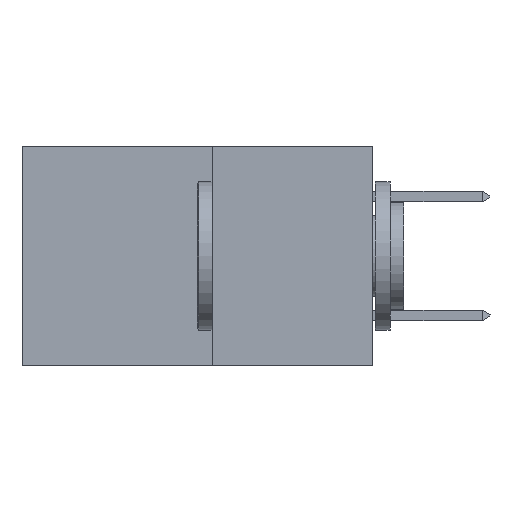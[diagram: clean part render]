
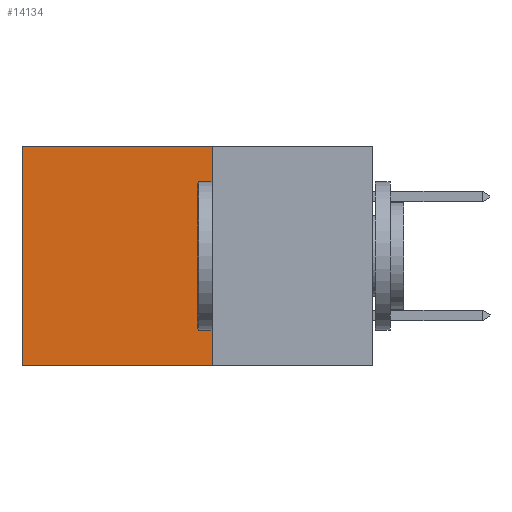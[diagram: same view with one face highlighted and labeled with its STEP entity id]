
A CAD part, left-side view. The second image highlights one B-rep face of the part: STEP entity #14134.
In plain terms, the highlighted planar face has unit normal (-1, 0, 0).
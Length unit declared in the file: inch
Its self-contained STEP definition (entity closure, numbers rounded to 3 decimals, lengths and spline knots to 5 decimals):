
#469 = EDGE_LOOP ( 'NONE', ( #17159, #15991, #15675, #19492 ) ) ;
#588 = EDGE_CURVE ( 'NONE', #6315, #1930, #10557, .T. ) ;
#1930 = VERTEX_POINT ( 'NONE', #6053 ) ;
#3744 = DIRECTION ( 'NONE',  ( 1., 0., 0. ) ) ;
#4343 = VERTEX_POINT ( 'NONE', #8386 ) ;
#6053 = CARTESIAN_POINT ( 'NONE',  ( 0.277, 0.59, 0. ) ) ;
#6055 = VECTOR ( 'NONE', #16469, 39.37008 ) ;
#6247 = EDGE_CURVE ( 'NONE', #1930, #4343, #13779, .T. ) ;
#6263 = EDGE_CURVE ( 'NONE', #6315, #13276, #17851, .T. ) ;
#6315 = VERTEX_POINT ( 'NONE', #9423 ) ;
#6545 = CARTESIAN_POINT ( 'NONE',  ( 0.277, 0.27, -0.37 ) ) ;
#6549 = EDGE_CURVE ( 'NONE', #13276, #4343, #12422, .T. ) ;
#6654 = DIRECTION ( 'NONE',  ( 0., 1., 0. ) ) ;
#8386 = CARTESIAN_POINT ( 'NONE',  ( 0.277, 0.59, -0.37 ) ) ;
#9423 = CARTESIAN_POINT ( 'NONE',  ( 0.277, 0.27, 0. ) ) ;
#9669 = DIRECTION ( 'NONE',  ( 0., 0., -1. ) ) ;
#9693 = CARTESIAN_POINT ( 'NONE',  ( 0.277, 0.27, -0.37 ) ) ;
#9844 = DIRECTION ( 'NONE',  ( 0., 0., -1. ) ) ;
#10080 = CARTESIAN_POINT ( 'NONE',  ( 0.277, 0.59, -0.37 ) ) ;
#10510 = PLANE ( 'NONE',  #16468 ) ;
#10557 = LINE ( 'NONE', #21573, #6055 ) ;
#12422 = LINE ( 'NONE', #6545, #17047 ) ;
#12696 = CARTESIAN_POINT ( 'NONE',  ( 0.277, 0.27, -0.37 ) ) ;
#13234 = VECTOR ( 'NONE', #9844, 39.37008 ) ;
#13276 = VERTEX_POINT ( 'NONE', #12696 ) ;
#13779 = LINE ( 'NONE', #10080, #13234 ) ;
#13925 = CARTESIAN_POINT ( 'NONE',  ( 0.277, 0.27, -0.37 ) ) ;
#14134 = ADVANCED_FACE ( 'NONE', ( #14988 ), #10510, .F. ) ;
#14988 = FACE_OUTER_BOUND ( 'NONE', #469, .T. ) ;
#15675 = ORIENTED_EDGE ( 'NONE', *, *, #6263, .F. ) ;
#15685 = DIRECTION ( 'NONE',  ( 0., 0., -1. ) ) ;
#15991 = ORIENTED_EDGE ( 'NONE', *, *, #6549, .F. ) ;
#16468 = AXIS2_PLACEMENT_3D ( 'NONE', #13925, #3744, #15685 ) ;
#16469 = DIRECTION ( 'NONE',  ( 0., 1., 0. ) ) ;
#17047 = VECTOR ( 'NONE', #6654, 39.37008 ) ;
#17159 = ORIENTED_EDGE ( 'NONE', *, *, #6247, .T. ) ;
#17851 = LINE ( 'NONE', #9693, #21795 ) ;
#19492 = ORIENTED_EDGE ( 'NONE', *, *, #588, .T. ) ;
#21573 = CARTESIAN_POINT ( 'NONE',  ( 0.277, 0.27, 0. ) ) ;
#21795 = VECTOR ( 'NONE', #9669, 39.37008 ) ;
